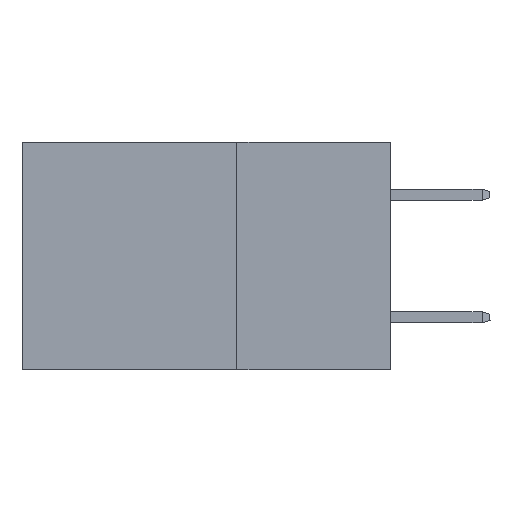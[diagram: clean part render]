
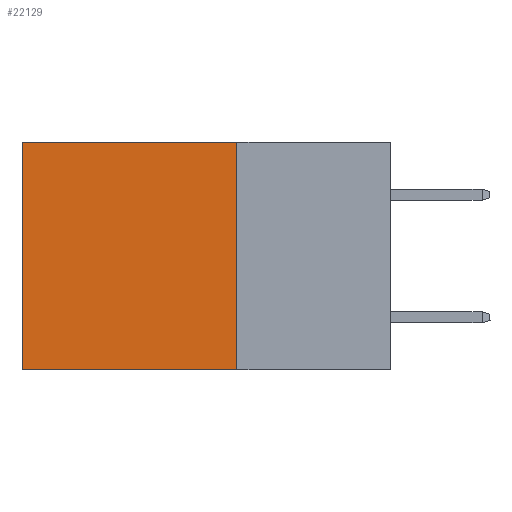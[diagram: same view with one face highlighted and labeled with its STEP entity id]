
A CAD part, left-side view. The second image highlights one B-rep face of the part: STEP entity #22129.
In plain terms, the highlighted planar face has unit normal (-1, 0, 0).
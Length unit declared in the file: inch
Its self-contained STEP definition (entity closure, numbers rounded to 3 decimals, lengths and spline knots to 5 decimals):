
#140 = VECTOR ( 'NONE', #18456, 39.37008 ) ;
#510 = VECTOR ( 'NONE', #1162, 39.37008 ) ;
#878 = CARTESIAN_POINT ( 'NONE',  ( 0.2875, 0.25, 0. ) ) ;
#1162 = DIRECTION ( 'NONE',  ( 0., 0., -1. ) ) ;
#1412 = DIRECTION ( 'NONE',  ( 0., 0., -1. ) ) ;
#3314 = CARTESIAN_POINT ( 'NONE',  ( 0.2875, 0.25, 0. ) ) ;
#3438 = VERTEX_POINT ( 'NONE', #11224 ) ;
#5779 = EDGE_CURVE ( 'NONE', #16353, #15186, #8268, .T. ) ;
#6754 = EDGE_CURVE ( 'NONE', #16353, #3438, #13438, .T. ) ;
#6774 = CARTESIAN_POINT ( 'NONE',  ( 0.2875, 0.25, -0.37 ) ) ;
#8268 = LINE ( 'NONE', #21997, #18375 ) ;
#10123 = EDGE_LOOP ( 'NONE', ( #21259, #18827, #14691, #23660 ) ) ;
#11224 = CARTESIAN_POINT ( 'NONE',  ( 0.2875, 0.25, -0.37 ) ) ;
#12037 = EDGE_CURVE ( 'NONE', #3438, #16796, #15446, .T. ) ;
#13438 = LINE ( 'NONE', #3314, #19839 ) ;
#13526 = AXIS2_PLACEMENT_3D ( 'NONE', #14562, #22444, #18543 ) ;
#14562 = CARTESIAN_POINT ( 'NONE',  ( 0.2875, 0.25, 0. ) ) ;
#14691 = ORIENTED_EDGE ( 'NONE', *, *, #6754, .F. ) ;
#15186 = VERTEX_POINT ( 'NONE', #21059 ) ;
#15446 = LINE ( 'NONE', #6774, #140 ) ;
#16353 = VERTEX_POINT ( 'NONE', #878 ) ;
#16563 = PLANE ( 'NONE',  #13526 ) ;
#16796 = VERTEX_POINT ( 'NONE', #18055 ) ;
#17298 = LINE ( 'NONE', #24602, #510 ) ;
#17454 = FACE_OUTER_BOUND ( 'NONE', #10123, .T. ) ;
#18055 = CARTESIAN_POINT ( 'NONE',  ( 0.2875, 0.6, -0.37 ) ) ;
#18375 = VECTOR ( 'NONE', #22257, 39.37008 ) ;
#18456 = DIRECTION ( 'NONE',  ( 0., 1., 0. ) ) ;
#18543 = DIRECTION ( 'NONE',  ( 0., 0., -1. ) ) ;
#18827 = ORIENTED_EDGE ( 'NONE', *, *, #12037, .F. ) ;
#19839 = VECTOR ( 'NONE', #1412, 39.37008 ) ;
#20927 = EDGE_CURVE ( 'NONE', #15186, #16796, #17298, .T. ) ;
#21059 = CARTESIAN_POINT ( 'NONE',  ( 0.2875, 0.6, 0. ) ) ;
#21259 = ORIENTED_EDGE ( 'NONE', *, *, #20927, .T. ) ;
#21997 = CARTESIAN_POINT ( 'NONE',  ( 0.2875, 0.25, 0. ) ) ;
#22129 = ADVANCED_FACE ( 'NONE', ( #17454 ), #16563, .F. ) ;
#22257 = DIRECTION ( 'NONE',  ( 0., 1., 0. ) ) ;
#22444 = DIRECTION ( 'NONE',  ( 1., 0., 0. ) ) ;
#23660 = ORIENTED_EDGE ( 'NONE', *, *, #5779, .T. ) ;
#24602 = CARTESIAN_POINT ( 'NONE',  ( 0.2875, 0.6, 0. ) ) ;
